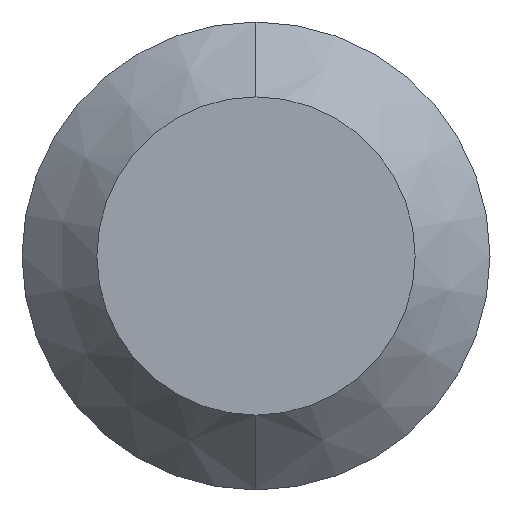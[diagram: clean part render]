
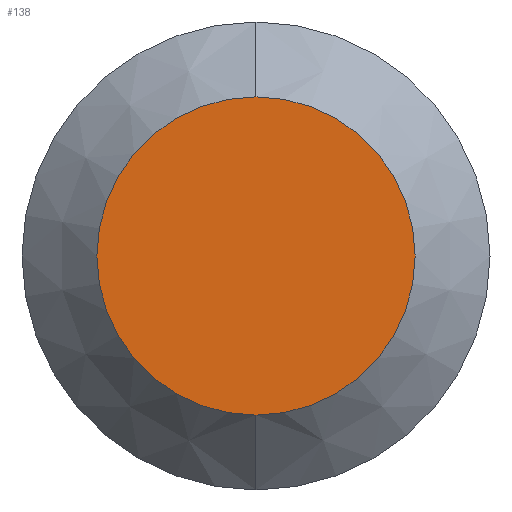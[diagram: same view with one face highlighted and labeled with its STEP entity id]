
A CAD part, left-side view. The second image highlights one B-rep face of the part: STEP entity #138.
In plain terms, the highlighted planar face has unit normal (-1, 0, 0).
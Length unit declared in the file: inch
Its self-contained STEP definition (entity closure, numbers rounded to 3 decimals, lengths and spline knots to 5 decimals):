
#4 = DIRECTION ( 'NONE',  ( 0., 0., -1. ) ) ;
#5 = DIRECTION ( 'NONE',  ( -1., 0., 0. ) ) ;
#18 = EDGE_LOOP ( 'NONE', ( #98, #236 ) ) ;
#19 = CARTESIAN_POINT ( 'NONE',  ( 0., 0., 0. ) ) ;
#28 = CIRCLE ( 'NONE', #80, 0.0425 ) ;
#52 = DIRECTION ( 'NONE',  ( 0., 0., -1. ) ) ;
#75 = DIRECTION ( 'NONE',  ( -1., 0., 0. ) ) ;
#76 = CARTESIAN_POINT ( 'NONE',  ( 0., 0., 0. ) ) ;
#78 = CARTESIAN_POINT ( 'NONE',  ( 0., 0., -0.0425 ) ) ;
#80 = AXIS2_PLACEMENT_3D ( 'NONE', #76, #75, #52 ) ;
#98 = ORIENTED_EDGE ( 'NONE', *, *, #188, .T. ) ;
#99 = DIRECTION ( 'NONE',  ( 0., 0., -1. ) ) ;
#100 = AXIS2_PLACEMENT_3D ( 'NONE', #19, #5, #4 ) ;
#101 = DIRECTION ( 'NONE',  ( 1., 0., 0. ) ) ;
#103 = AXIS2_PLACEMENT_3D ( 'NONE', #118, #101, #99 ) ;
#114 = PLANE ( 'NONE',  #103 ) ;
#118 = CARTESIAN_POINT ( 'NONE',  ( 0., 0., 0. ) ) ;
#138 = ADVANCED_FACE ( 'NONE', ( #189 ), #114, .F. ) ;
#149 = EDGE_CURVE ( 'NONE', #198, #204, #226, .T. ) ;
#161 = CARTESIAN_POINT ( 'NONE',  ( 0., 0., 0.0425 ) ) ;
#188 = EDGE_CURVE ( 'NONE', #204, #198, #28, .T. ) ;
#189 = FACE_OUTER_BOUND ( 'NONE', #18, .T. ) ;
#198 = VERTEX_POINT ( 'NONE', #161 ) ;
#204 = VERTEX_POINT ( 'NONE', #78 ) ;
#226 = CIRCLE ( 'NONE', #100, 0.0425 ) ;
#236 = ORIENTED_EDGE ( 'NONE', *, *, #149, .T. ) ;
